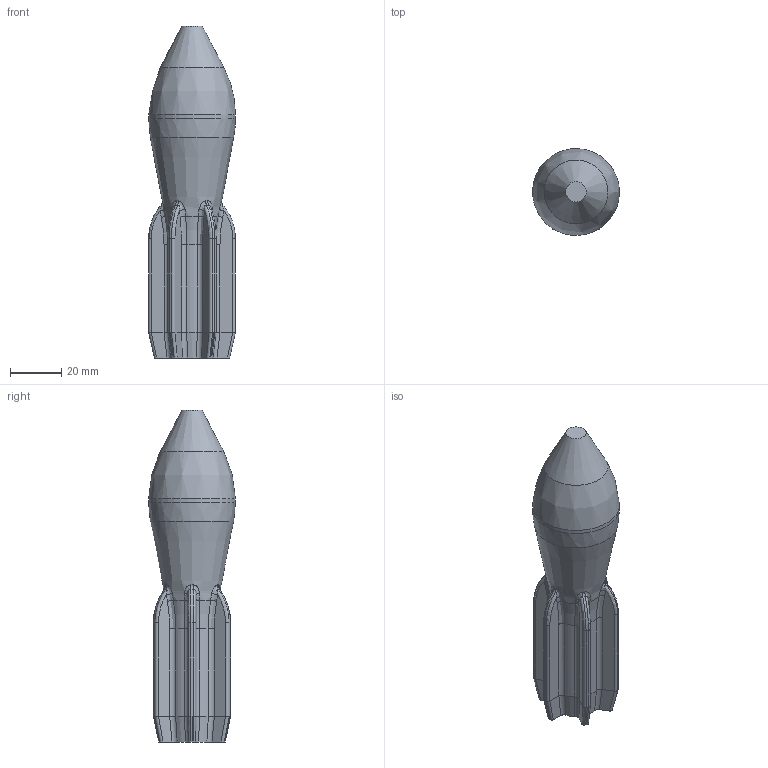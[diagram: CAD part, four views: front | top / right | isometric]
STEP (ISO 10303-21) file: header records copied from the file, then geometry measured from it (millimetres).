
FILE_DESCRIPTION(('FreeCAD Model'),'2;1');
FILE_NAME('Open CASCADE Shape Model','2022-10-05T16:36:22',('Author'),( ''),'Open CASCADE STEP processor 7.6','FreeCAD','Unknown');
FILE_SCHEMA(('AUTOMOTIVE_DESIGN { 1 0 10303 214 1 1 1 1 }'));
Length unit declared in the file: millimetre
Products named in the file (1): Projectile
Bounding box: 34 x 33.97 x 129.99 mm (x, y, z)
Volume: 66755.6 mm3; surface area: 14486.6 mm2
Topology: 1 solids, 1 shells, 176 faces, 409 edges, 235 vertices
Faces by surface type: bspline 99, cylinder 37, plane 20, torus 12, cone 8
Full cylindrical faces by diameter (mm): 34 x1
Entity records: 22497 total; most frequent: CARTESIAN_POINT 15730, DIRECTION 835, ORIENTED_EDGE 818, PCURVE 818, DEFINITIONAL_REPRESENTATION 818, LINE 514, VECTOR 514, B_SPLINE_CURVE_WITH_KNOTS 468
